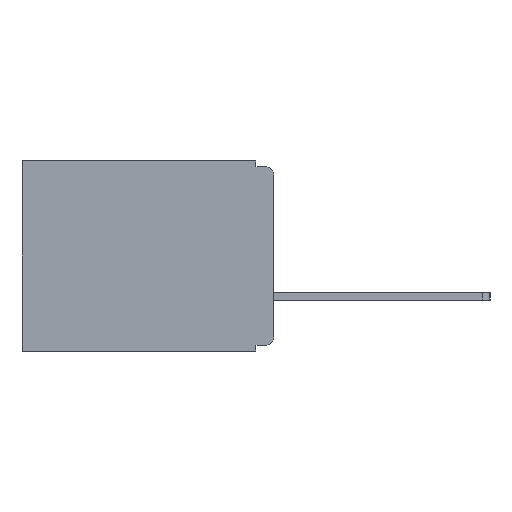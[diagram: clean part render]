
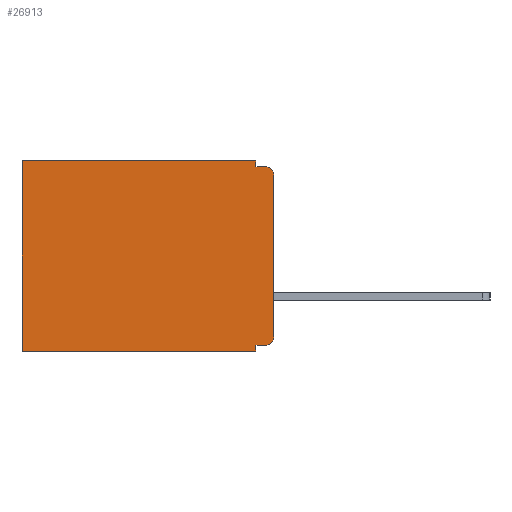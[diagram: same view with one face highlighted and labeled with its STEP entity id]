
A CAD part, left-side view. The second image highlights one B-rep face of the part: STEP entity #26913.
In plain terms, the highlighted planar face has unit normal (-1, 0, 0).
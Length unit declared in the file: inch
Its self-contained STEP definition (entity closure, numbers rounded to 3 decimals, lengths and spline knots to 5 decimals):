
#94 = VERTEX_POINT ( 'NONE', #1213 ) ;
#141 = DIRECTION ( 'NONE',  ( 0., 1., 0. ) ) ;
#1213 = CARTESIAN_POINT ( 'NONE',  ( 0.3, 0.437, -0.33 ) ) ;
#1445 = DIRECTION ( 'NONE',  ( -1., 0., 0. ) ) ;
#1447 = CARTESIAN_POINT ( 'NONE',  ( 0.3, 0.031, -0.32 ) ) ;
#1787 = ORIENTED_EDGE ( 'NONE', *, *, #19217, .T. ) ;
#1909 = LINE ( 'NONE', #23930, #18639 ) ;
#2162 = EDGE_CURVE ( 'NONE', #17355, #94, #26596, .T. ) ;
#2236 = DIRECTION ( 'NONE',  ( 0., 0., -1. ) ) ;
#2603 = CARTESIAN_POINT ( 'NONE',  ( 0.3, 0.031, 0. ) ) ;
#2638 = DIRECTION ( 'NONE',  ( 0., 0., -1. ) ) ;
#2854 = VERTEX_POINT ( 'NONE', #14123 ) ;
#3179 = ORIENTED_EDGE ( 'NONE', *, *, #3384, .F. ) ;
#3384 = EDGE_CURVE ( 'NONE', #29867, #6134, #11596, .T. ) ;
#3768 = EDGE_CURVE ( 'NONE', #7389, #21348, #8200, .T. ) ;
#4376 = CARTESIAN_POINT ( 'NONE',  ( 0.3, 0.437, 0. ) ) ;
#4903 = LINE ( 'NONE', #16658, #16834 ) ;
#5082 = DIRECTION ( 'NONE',  ( 0., 0., -1. ) ) ;
#5179 = VECTOR ( 'NONE', #8253, 39.37008 ) ;
#5438 = CARTESIAN_POINT ( 'NONE',  ( 0.3, 0., 0. ) ) ;
#6134 = VERTEX_POINT ( 'NONE', #12980 ) ;
#7389 = VERTEX_POINT ( 'NONE', #30046 ) ;
#7768 = CARTESIAN_POINT ( 'NONE',  ( 0.3, 0.031, -0.33 ) ) ;
#7866 = DIRECTION ( 'NONE',  ( -1., 0., 0. ) ) ;
#7885 = DIRECTION ( 'NONE',  ( 0., 1., 0. ) ) ;
#8200 = CIRCLE ( 'NONE', #26857, 0.015 ) ;
#8253 = DIRECTION ( 'NONE',  ( 0., -1., 0. ) ) ;
#8464 = ORIENTED_EDGE ( 'NONE', *, *, #12122, .F. ) ;
#9312 = VECTOR ( 'NONE', #17662, 39.37008 ) ;
#9497 = ORIENTED_EDGE ( 'NONE', *, *, #3768, .T. ) ;
#10478 = DIRECTION ( 'NONE',  ( 1., 0., 0. ) ) ;
#11596 = LINE ( 'NONE', #24316, #5179 ) ;
#12067 = EDGE_CURVE ( 'NONE', #7389, #12393, #4903, .T. ) ;
#12122 = EDGE_CURVE ( 'NONE', #15360, #29867, #16116, .T. ) ;
#12393 = VERTEX_POINT ( 'NONE', #1447 ) ;
#12955 = CARTESIAN_POINT ( 'NONE',  ( 0.3, 0., -0.33 ) ) ;
#12980 = CARTESIAN_POINT ( 'NONE',  ( 0.3, 0.015, -0.01 ) ) ;
#13337 = EDGE_CURVE ( 'NONE', #12393, #17355, #1909, .T. ) ;
#13773 = DIRECTION ( 'NONE',  ( 0., 1., 0. ) ) ;
#14021 = CARTESIAN_POINT ( 'NONE',  ( 0.3, 0., -0.33 ) ) ;
#14123 = CARTESIAN_POINT ( 'NONE',  ( 0.3, 0., -0.025 ) ) ;
#14659 = EDGE_LOOP ( 'NONE', ( #16290, #19813, #3179, #8464, #1787, #25113, #20050, #23990, #20910, #9497 ) ) ;
#14986 = VECTOR ( 'NONE', #13773, 39.37008 ) ;
#15360 = VERTEX_POINT ( 'NONE', #30248 ) ;
#15728 = CARTESIAN_POINT ( 'NONE',  ( 0.3, 0.015, -0.025 ) ) ;
#15783 = VECTOR ( 'NONE', #7885, 39.37008 ) ;
#15887 = CARTESIAN_POINT ( 'NONE',  ( 0.3, 0.015, -0.305 ) ) ;
#16116 = LINE ( 'NONE', #2603, #28333 ) ;
#16167 = LINE ( 'NONE', #18866, #27700 ) ;
#16290 = ORIENTED_EDGE ( 'NONE', *, *, #27586, .F. ) ;
#16658 = CARTESIAN_POINT ( 'NONE',  ( 0.3, 0., -0.32 ) ) ;
#16834 = VECTOR ( 'NONE', #141, 39.37008 ) ;
#17355 = VERTEX_POINT ( 'NONE', #7768 ) ;
#17662 = DIRECTION ( 'NONE',  ( 0., 0., -1. ) ) ;
#18075 = DIRECTION ( 'NONE',  ( 0., 0., -1. ) ) ;
#18639 = VECTOR ( 'NONE', #2638, 39.37008 ) ;
#18866 = CARTESIAN_POINT ( 'NONE',  ( 0.3, 0.437, -0.33 ) ) ;
#18977 = DIRECTION ( 'NONE',  ( 0., 0., -1. ) ) ;
#19038 = EDGE_CURVE ( 'NONE', #29525, #94, #16167, .T. ) ;
#19217 = EDGE_CURVE ( 'NONE', #15360, #29525, #21983, .T. ) ;
#19813 = ORIENTED_EDGE ( 'NONE', *, *, #29899, .T. ) ;
#19841 = PLANE ( 'NONE',  #26357 ) ;
#20050 = ORIENTED_EDGE ( 'NONE', *, *, #2162, .F. ) ;
#20910 = ORIENTED_EDGE ( 'NONE', *, *, #12067, .F. ) ;
#21348 = VERTEX_POINT ( 'NONE', #28667 ) ;
#21828 = LINE ( 'NONE', #12955, #9312 ) ;
#21983 = LINE ( 'NONE', #5438, #15783 ) ;
#22993 = FACE_OUTER_BOUND ( 'NONE', #14659, .T. ) ;
#23930 = CARTESIAN_POINT ( 'NONE',  ( 0.3, 0.031, -0.33 ) ) ;
#23990 = ORIENTED_EDGE ( 'NONE', *, *, #13337, .F. ) ;
#24316 = CARTESIAN_POINT ( 'NONE',  ( 0.3, 0., -0.01 ) ) ;
#25113 = ORIENTED_EDGE ( 'NONE', *, *, #19038, .T. ) ;
#26218 = AXIS2_PLACEMENT_3D ( 'NONE', #15728, #1445, #18075 ) ;
#26357 = AXIS2_PLACEMENT_3D ( 'NONE', #26688, #10478, #26773 ) ;
#26596 = LINE ( 'NONE', #14021, #14986 ) ;
#26688 = CARTESIAN_POINT ( 'NONE',  ( 0.3, 0., -0.33 ) ) ;
#26773 = DIRECTION ( 'NONE',  ( 0., 0., -1. ) ) ;
#26857 = AXIS2_PLACEMENT_3D ( 'NONE', #15887, #7866, #18977 ) ;
#26913 = ADVANCED_FACE ( 'NONE', ( #22993 ), #19841, .F. ) ;
#27586 = EDGE_CURVE ( 'NONE', #2854, #21348, #21828, .T. ) ;
#27700 = VECTOR ( 'NONE', #2236, 39.37008 ) ;
#28333 = VECTOR ( 'NONE', #5082, 39.37008 ) ;
#28667 = CARTESIAN_POINT ( 'NONE',  ( 0.3, 0., -0.305 ) ) ;
#28716 = CIRCLE ( 'NONE', #26218, 0.015 ) ;
#29308 = CARTESIAN_POINT ( 'NONE',  ( 0.3, 0.031, -0.01 ) ) ;
#29525 = VERTEX_POINT ( 'NONE', #4376 ) ;
#29867 = VERTEX_POINT ( 'NONE', #29308 ) ;
#29899 = EDGE_CURVE ( 'NONE', #2854, #6134, #28716, .T. ) ;
#30046 = CARTESIAN_POINT ( 'NONE',  ( 0.3, 0.015, -0.32 ) ) ;
#30248 = CARTESIAN_POINT ( 'NONE',  ( 0.3, 0.031, 0. ) ) ;
